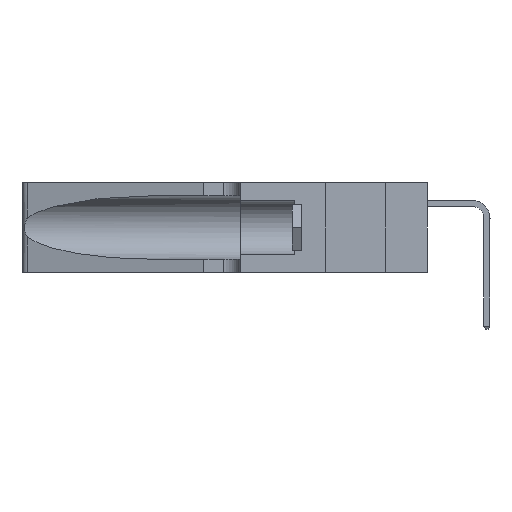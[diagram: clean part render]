
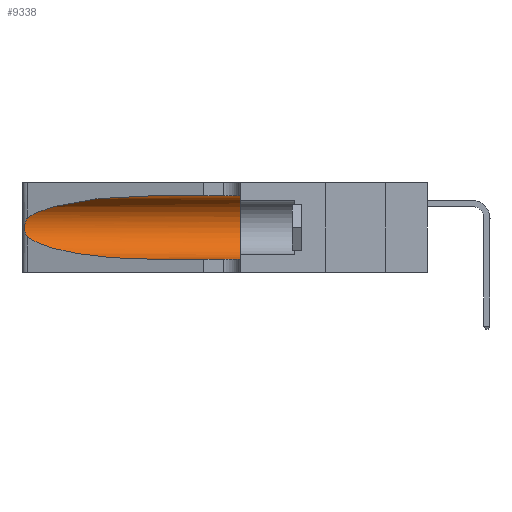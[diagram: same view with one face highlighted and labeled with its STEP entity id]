
A CAD part, left-side view. The second image highlights one B-rep face of the part: STEP entity #9338.
In plain terms, the highlighted cylindrical face has radius 3.308 mm (diameter 6.617 mm), a partial arc.
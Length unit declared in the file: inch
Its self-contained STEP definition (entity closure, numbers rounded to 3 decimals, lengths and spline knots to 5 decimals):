
#111 = CARTESIAN_POINT ( 'NONE',  ( 0.1305, 0.72297, 0.31525 ) ) ;
#658 = CARTESIAN_POINT ( 'NONE',  ( 0.1305, 0.35, 0.31525 ) ) ;
#1856 = CARTESIAN_POINT ( 'NONE',  ( 0.25487, 1.22718, 0.22369 ) ) ;
#1967 = EDGE_CURVE ( 'NONE', #17580, #17910, #18477, .T. ) ;
#2429 = CARTESIAN_POINT ( 'NONE',  ( 0.25639, 1.23186, 0.15144 ) ) ;
#4952 = VECTOR ( 'NONE', #25084, 39.37008 ) ;
#5634 = CARTESIAN_POINT ( 'NONE',  ( 0.25487, 1.22718, 0.14631 ) ) ;
#6455 = CARTESIAN_POINT ( 'NONE',  ( 0.25487, 1.22718, 0.14631 ) ) ;
#6834 = AXIS2_PLACEMENT_3D ( 'NONE', #15562, #19623, #23683 ) ;
#7235 = LINE ( 'NONE', #38343, #38052 ) ;
#9338 = ADVANCED_FACE ( 'NONE', ( #37353 ), #45423, .F. ) ;
#9788 = CARTESIAN_POINT ( 'NONE',  ( 0.1305, 0.72297, 0.31525 ) ) ;
#10367 = CARTESIAN_POINT ( 'NONE',  ( 0.25639, 1.23184, 0.21858 ) ) ;
#13284 = DIRECTION ( 'NONE',  ( 0., 1., 0. ) ) ;
#14403 = EDGE_CURVE ( 'NONE', #17910, #22410, #46348, .T. ) ;
#14439 = CARTESIAN_POINT ( 'NONE',  ( 0.25854, 1.2359, 0.20912 ) ) ;
#15562 = CARTESIAN_POINT ( 'NONE',  ( 0.1305, 1.61858, 0.185 ) ) ;
#15940 = ORIENTED_EDGE ( 'NONE', *, *, #39417, .T. ) ;
#15957 = CARTESIAN_POINT ( 'NONE',  ( 0.25487, 1.22718, 0.14631 ) ) ;
#17580 = VERTEX_POINT ( 'NONE', #5634 ) ;
#17614 = CARTESIAN_POINT ( 'NONE',  ( 0.25487, 1.22718, 0.22369 ) ) ;
#17910 = VERTEX_POINT ( 'NONE', #32569 ) ;
#18312 = CARTESIAN_POINT ( 'NONE',  ( 0.25555, 1.22994, 0.2215 ) ) ;
#18477 =( BOUNDED_CURVE ( )  B_SPLINE_CURVE ( 3, ( #15957, #39944, #35954, #43936 ),
 .UNSPECIFIED., .F., .T. ) 
 B_SPLINE_CURVE_WITH_KNOTS ( ( 4, 4 ),
 ( 3.44316, 4.71239 ),
 .UNSPECIFIED. ) 
 CURVE ( )  GEOMETRIC_REPRESENTATION_ITEM ( )  RATIONAL_B_SPLINE_CURVE ( ( 1., 0.87, 0.87, 1. ) ) 
 REPRESENTATION_ITEM ( '' )  );
#18484 = CARTESIAN_POINT ( 'NONE',  ( 0.26075, 1.23896, 0.19203 ) ) ;
#19623 = DIRECTION ( 'NONE',  ( 0., -1., 0. ) ) ;
#20651 = CIRCLE ( 'NONE', #35969, 0.13025 ) ;
#22132 = ORIENTED_EDGE ( 'NONE', *, *, #1967, .T. ) ;
#22410 = VERTEX_POINT ( 'NONE', #22869 ) ;
#22549 = CARTESIAN_POINT ( 'NONE',  ( 0.26017, 1.23833, 0.17102 ) ) ;
#22869 = CARTESIAN_POINT ( 'NONE',  ( 0.1305, 0.35, 0.05475 ) ) ;
#23683 = DIRECTION ( 'NONE',  ( 0., 0., -1. ) ) ;
#24165 = EDGE_LOOP ( 'NONE', ( #15940, #31134, #22132, #45672, #51324, #47672 ) ) ;
#25084 = DIRECTION ( 'NONE',  ( 0., -1., 0. ) ) ;
#25278 = VERTEX_POINT ( 'NONE', #17614 ) ;
#26069 = CARTESIAN_POINT ( 'NONE',  ( 0.2373, 1.15595, 0.28018 ) ) ;
#26453 = CARTESIAN_POINT ( 'NONE',  ( 0.25487, 1.22718, 0.22369 ) ) ;
#26624 = CARTESIAN_POINT ( 'NONE',  ( 0.25789, 1.23486, 0.15765 ) ) ;
#29111 = CARTESIAN_POINT ( 'NONE',  ( 0.1305, 1.61858, 0.05475 ) ) ;
#29468 = B_SPLINE_CURVE_WITH_KNOTS ( 'NONE', 3,
 ( #26453, #18312, #10367, #38445, #14439, #42455, #18484, #46433, #22549, #50400, #26624, #2429, #30614, #6455 ),
 .UNSPECIFIED., .F., .F.,
 ( 4, 2, 2, 2, 2, 2, 4 ),
 ( 0., 0.00027, 0.00053, 0.00107, 0.0016, 0.00187, 0.00214 ),
 .UNSPECIFIED. ) ;
#30614 = CARTESIAN_POINT ( 'NONE',  ( 0.25555, 1.22993, 0.14849 ) ) ;
#30826 = VERTEX_POINT ( 'NONE', #111 ) ;
#31134 = ORIENTED_EDGE ( 'NONE', *, *, #41633, .T. ) ;
#32569 = CARTESIAN_POINT ( 'NONE',  ( 0.1305, 0.72297, 0.05475 ) ) ;
#32659 = EDGE_CURVE ( 'NONE', #30826, #44066, #7235, .T. ) ;
#35954 = CARTESIAN_POINT ( 'NONE',  ( 0.18966, 0.96281, 0.05475 ) ) ;
#35969 = AXIS2_PLACEMENT_3D ( 'NONE', #37310, #13284, #41301 ) ;
#37310 = CARTESIAN_POINT ( 'NONE',  ( 0.1305, 0.35, 0.185 ) ) ;
#37353 = FACE_OUTER_BOUND ( 'NONE', #24165, .T. ) ;
#38052 = VECTOR ( 'NONE', #42347, 39.37008 ) ;
#38343 = CARTESIAN_POINT ( 'NONE',  ( 0.1305, 1.61858, 0.31525 ) ) ;
#38445 = CARTESIAN_POINT ( 'NONE',  ( 0.25787, 1.23484, 0.2124 ) ) ;
#39417 = EDGE_CURVE ( 'NONE', #30826, #25278, #47916, .T. ) ;
#39944 = CARTESIAN_POINT ( 'NONE',  ( 0.2373, 1.15595, 0.08982 ) ) ;
#39959 = EDGE_CURVE ( 'NONE', #44066, #22410, #20651, .T. ) ;
#41301 = DIRECTION ( 'NONE',  ( 0., 0., 1. ) ) ;
#41633 = EDGE_CURVE ( 'NONE', #25278, #17580, #29468, .T. ) ;
#42347 = DIRECTION ( 'NONE',  ( 0., -1., 0. ) ) ;
#42455 = CARTESIAN_POINT ( 'NONE',  ( 0.26018, 1.23835, 0.19895 ) ) ;
#43936 = CARTESIAN_POINT ( 'NONE',  ( 0.1305, 0.72297, 0.05475 ) ) ;
#44066 = VERTEX_POINT ( 'NONE', #658 ) ;
#45423 = CYLINDRICAL_SURFACE ( 'NONE', #6834, 0.13025 ) ;
#45672 = ORIENTED_EDGE ( 'NONE', *, *, #14403, .T. ) ;
#45881 = CARTESIAN_POINT ( 'NONE',  ( 0.18966, 0.96281, 0.31525 ) ) ;
#46348 = LINE ( 'NONE', #29111, #4952 ) ;
#46433 = CARTESIAN_POINT ( 'NONE',  ( 0.26075, 1.23896, 0.178 ) ) ;
#47672 = ORIENTED_EDGE ( 'NONE', *, *, #32659, .F. ) ;
#47916 =( BOUNDED_CURVE ( )  B_SPLINE_CURVE ( 3, ( #9788, #45881, #26069, #1856 ),
 .UNSPECIFIED., .F., .F. ) 
 B_SPLINE_CURVE_WITH_KNOTS ( ( 4, 4 ),
 ( 1.5708, 2.84003 ),
 .UNSPECIFIED. ) 
 CURVE ( )  GEOMETRIC_REPRESENTATION_ITEM ( )  RATIONAL_B_SPLINE_CURVE ( ( 1., 0.87, 0.87, 1. ) ) 
 REPRESENTATION_ITEM ( '' )  );
#50400 = CARTESIAN_POINT ( 'NONE',  ( 0.25856, 1.23593, 0.16098 ) ) ;
#51324 = ORIENTED_EDGE ( 'NONE', *, *, #39959, .F. ) ;
